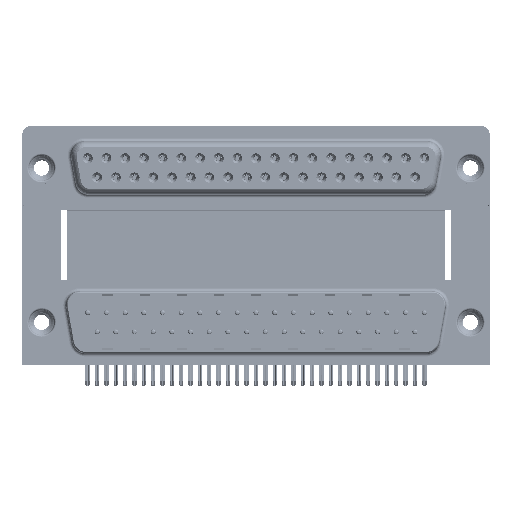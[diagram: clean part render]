
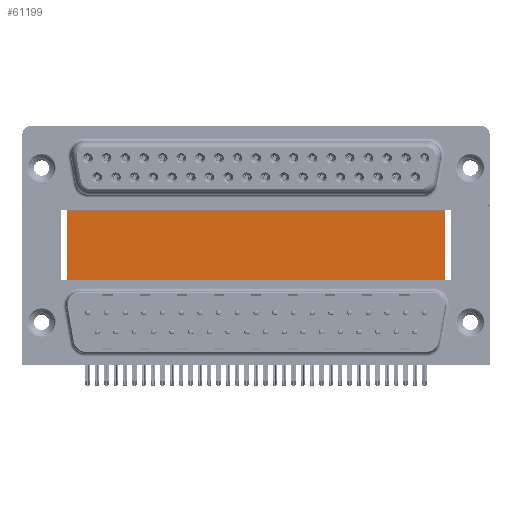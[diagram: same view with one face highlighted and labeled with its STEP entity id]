
A CAD part, top view. The second image highlights one B-rep face of the part: STEP entity #61199.
In plain terms, the highlighted planar face has unit normal (0, 0, 1).
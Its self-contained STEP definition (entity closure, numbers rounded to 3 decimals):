
#3420 = CARTESIAN_POINT ( 'NONE',  ( 3.79, 16.585, -12. ) ) ;
#4251 = EDGE_CURVE ( 'NONE', #24205, #17458, #22939, .T. ) ;
#5001 = DIRECTION ( 'NONE',  ( 1., 0., 0. ) ) ;
#13513 = CARTESIAN_POINT ( 'NONE',  ( 3.79, -3.735, -12. ) ) ;
#16784 = CARTESIAN_POINT ( 'NONE',  ( 3.79, -3.735, -12. ) ) ;
#17458 = VERTEX_POINT ( 'NONE', #16784 ) ;
#22939 = LINE ( 'NONE', #23602, #43704 ) ;
#23602 = CARTESIAN_POINT ( 'NONE',  ( 3.79, 16.585, -12. ) ) ;
#24205 = VERTEX_POINT ( 'NONE', #48164 ) ;
#26282 = LINE ( 'NONE', #57370, #36181 ) ;
#26323 = FACE_OUTER_BOUND ( 'NONE', #44061, .T. ) ;
#27925 = DIRECTION ( 'NONE',  ( 1., 0., 0. ) ) ;
#30762 = DIRECTION ( 'NONE',  ( 0., 0., -1. ) ) ;
#32017 = EDGE_CURVE ( 'NONE', #24205, #51623, #26282, .T. ) ;
#33369 = ORIENTED_EDGE ( 'NONE', *, *, #57274, .T. ) ;
#35253 = LINE ( 'NONE', #45849, #40182 ) ;
#35904 = DIRECTION ( 'NONE',  ( -1., 0., 0. ) ) ;
#36181 = VECTOR ( 'NONE', #5001, 1000. ) ;
#36270 = CARTESIAN_POINT ( 'NONE',  ( 59.71, 16.585, -12. ) ) ;
#38447 = CARTESIAN_POINT ( 'NONE',  ( 59.71, -3.735, -12. ) ) ;
#40182 = VECTOR ( 'NONE', #61203, 1000. ) ;
#43704 = VECTOR ( 'NONE', #43804, 1000. ) ;
#43804 = DIRECTION ( 'NONE',  ( 0., -1., 0. ) ) ;
#44061 = EDGE_LOOP ( 'NONE', ( #33369, #64336, #44447, #52574 ) ) ;
#44447 = ORIENTED_EDGE ( 'NONE', *, *, #32017, .F. ) ;
#45849 = CARTESIAN_POINT ( 'NONE',  ( 59.71, 16.585, -12. ) ) ;
#48164 = CARTESIAN_POINT ( 'NONE',  ( 3.79, 16.585, -12. ) ) ;
#49040 = AXIS2_PLACEMENT_3D ( 'NONE', #3420, #30762, #35904 ) ;
#51623 = VERTEX_POINT ( 'NONE', #36270 ) ;
#52574 = ORIENTED_EDGE ( 'NONE', *, *, #4251, .T. ) ;
#54234 = LINE ( 'NONE', #13513, #56311 ) ;
#56311 = VECTOR ( 'NONE', #27925, 1000. ) ;
#57274 = EDGE_CURVE ( 'NONE', #17458, #58803, #54234, .T. ) ;
#57370 = CARTESIAN_POINT ( 'NONE',  ( 3.79, 16.585, -12. ) ) ;
#58803 = VERTEX_POINT ( 'NONE', #38447 ) ;
#59421 = EDGE_CURVE ( 'NONE', #51623, #58803, #35253, .T. ) ;
#61199 = ADVANCED_FACE ( 'NONE', ( #26323 ), #66047, .F. ) ;
#61203 = DIRECTION ( 'NONE',  ( 0., -1., 0. ) ) ;
#64336 = ORIENTED_EDGE ( 'NONE', *, *, #59421, .F. ) ;
#66047 = PLANE ( 'NONE',  #49040 ) ;
